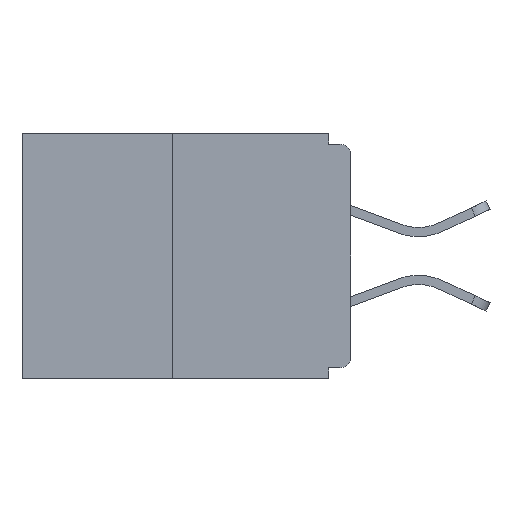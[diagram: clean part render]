
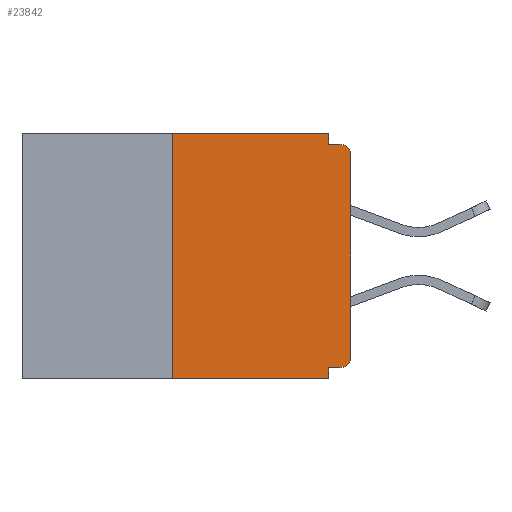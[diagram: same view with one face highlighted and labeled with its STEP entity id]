
A CAD part, left-side view. The second image highlights one B-rep face of the part: STEP entity #23842.
In plain terms, the highlighted planar face has unit normal (-1, 0, 0).
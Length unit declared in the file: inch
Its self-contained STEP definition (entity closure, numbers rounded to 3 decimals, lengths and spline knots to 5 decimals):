
#262 = CARTESIAN_POINT ( 'NONE',  ( 0., 0.015, -0.015 ) ) ;
#579 = CARTESIAN_POINT ( 'NONE',  ( 0., 0.015, -0.328 ) ) ;
#1026 = ORIENTED_EDGE ( 'NONE', *, *, #3591, .F. ) ;
#1222 = VERTEX_POINT ( 'NONE', #15468 ) ;
#1596 = LINE ( 'NONE', #5494, #14856 ) ;
#1816 = EDGE_LOOP ( 'NONE', ( #1026, #21679, #14848, #4472, #8057, #8399, #24403, #12604, #2949, #17886 ) ) ;
#2138 = CARTESIAN_POINT ( 'NONE',  ( 0., 0.031, -0.328 ) ) ;
#2423 = CIRCLE ( 'NONE', #19418, 0.015 ) ;
#2949 = ORIENTED_EDGE ( 'NONE', *, *, #5460, .F. ) ;
#3169 = AXIS2_PLACEMENT_3D ( 'NONE', #14497, #12615, #20066 ) ;
#3219 = CARTESIAN_POINT ( 'NONE',  ( 0., 0.031, -0.343 ) ) ;
#3417 = EDGE_CURVE ( 'NONE', #15087, #22866, #13087, .T. ) ;
#3517 = CARTESIAN_POINT ( 'NONE',  ( 0., 0.25, 0. ) ) ;
#3591 = EDGE_CURVE ( 'NONE', #1222, #23844, #17242, .T. ) ;
#3611 = DIRECTION ( 'NONE',  ( 0., -1., 0. ) ) ;
#3667 = LINE ( 'NONE', #18871, #14287 ) ;
#4472 = ORIENTED_EDGE ( 'NONE', *, *, #3417, .F. ) ;
#4633 = VECTOR ( 'NONE', #23234, 39.37008 ) ;
#5460 = EDGE_CURVE ( 'NONE', #10794, #6925, #3667, .T. ) ;
#5494 = CARTESIAN_POINT ( 'NONE',  ( 0., 0.46, -0.343 ) ) ;
#5943 = CARTESIAN_POINT ( 'NONE',  ( 0., 0.46, 0. ) ) ;
#6136 = VERTEX_POINT ( 'NONE', #579 ) ;
#6344 = EDGE_CURVE ( 'NONE', #21519, #23504, #22492, .T. ) ;
#6925 = VERTEX_POINT ( 'NONE', #262 ) ;
#7069 = EDGE_CURVE ( 'NONE', #23844, #10794, #14672, .T. ) ;
#7860 = CARTESIAN_POINT ( 'NONE',  ( 0., 0., 0. ) ) ;
#8057 = ORIENTED_EDGE ( 'NONE', *, *, #11581, .F. ) ;
#8399 = ORIENTED_EDGE ( 'NONE', *, *, #18187, .T. ) ;
#9705 = LINE ( 'NONE', #3517, #24571 ) ;
#9790 = CARTESIAN_POINT ( 'NONE',  ( 0., 0.031, -0.015 ) ) ;
#10006 = DIRECTION ( 'NONE',  ( -1., 0., 0. ) ) ;
#10794 = VERTEX_POINT ( 'NONE', #9790 ) ;
#11289 = VECTOR ( 'NONE', #23975, 39.37008 ) ;
#11453 = VECTOR ( 'NONE', #12535, 39.37008 ) ;
#11581 = EDGE_CURVE ( 'NONE', #6136, #15087, #17865, .T. ) ;
#11954 = CARTESIAN_POINT ( 'NONE',  ( 0., 0., -0.03 ) ) ;
#12359 = PLANE ( 'NONE',  #3169 ) ;
#12535 = DIRECTION ( 'NONE',  ( 0., 0., -1. ) ) ;
#12558 = DIRECTION ( 'NONE',  ( -1., 0., 0. ) ) ;
#12604 = ORIENTED_EDGE ( 'NONE', *, *, #18115, .T. ) ;
#12615 = DIRECTION ( 'NONE',  ( 1., 0., 0. ) ) ;
#13087 = LINE ( 'NONE', #22949, #11289 ) ;
#13827 = CARTESIAN_POINT ( 'NONE',  ( 0., 0.015, -0.03 ) ) ;
#13964 = CARTESIAN_POINT ( 'NONE',  ( 0., 0., -0.328 ) ) ;
#14156 = CIRCLE ( 'NONE', #23062, 0.015 ) ;
#14212 = EDGE_CURVE ( 'NONE', #14976, #22866, #1596, .T. ) ;
#14284 = CARTESIAN_POINT ( 'NONE',  ( 0., 0.031, 0. ) ) ;
#14287 = VECTOR ( 'NONE', #24703, 39.37008 ) ;
#14497 = CARTESIAN_POINT ( 'NONE',  ( 0., 0.46, 0. ) ) ;
#14571 = DIRECTION ( 'NONE',  ( 0., 0., -1. ) ) ;
#14672 = LINE ( 'NONE', #14284, #11453 ) ;
#14848 = ORIENTED_EDGE ( 'NONE', *, *, #14212, .T. ) ;
#14856 = VECTOR ( 'NONE', #3611, 39.37008 ) ;
#14976 = VERTEX_POINT ( 'NONE', #17101 ) ;
#15087 = VERTEX_POINT ( 'NONE', #2138 ) ;
#15255 = CARTESIAN_POINT ( 'NONE',  ( 0., 0., -0.313 ) ) ;
#15468 = CARTESIAN_POINT ( 'NONE',  ( 0., 0.25, 0. ) ) ;
#17101 = CARTESIAN_POINT ( 'NONE',  ( 0., 0.25, -0.343 ) ) ;
#17242 = LINE ( 'NONE', #5943, #21034 ) ;
#17865 = LINE ( 'NONE', #13964, #4633 ) ;
#17886 = ORIENTED_EDGE ( 'NONE', *, *, #7069, .F. ) ;
#18115 = EDGE_CURVE ( 'NONE', #23504, #6925, #2423, .T. ) ;
#18187 = EDGE_CURVE ( 'NONE', #6136, #21519, #14156, .T. ) ;
#18562 = DIRECTION ( 'NONE',  ( 0., 0., 1. ) ) ;
#18871 = CARTESIAN_POINT ( 'NONE',  ( 0., 0., -0.015 ) ) ;
#19086 = DIRECTION ( 'NONE',  ( 0., 0., 1. ) ) ;
#19161 = VECTOR ( 'NONE', #18562, 39.37008 ) ;
#19400 = DIRECTION ( 'NONE',  ( 0., -1., 0. ) ) ;
#19418 = AXIS2_PLACEMENT_3D ( 'NONE', #13827, #10006, #21788 ) ;
#20066 = DIRECTION ( 'NONE',  ( 0., 0., -1. ) ) ;
#20333 = CARTESIAN_POINT ( 'NONE',  ( 0., 0.031, 0. ) ) ;
#21034 = VECTOR ( 'NONE', #19400, 39.37008 ) ;
#21519 = VERTEX_POINT ( 'NONE', #15255 ) ;
#21679 = ORIENTED_EDGE ( 'NONE', *, *, #24797, .F. ) ;
#21788 = DIRECTION ( 'NONE',  ( 0., 0., -1. ) ) ;
#21974 = FACE_OUTER_BOUND ( 'NONE', #1816, .T. ) ;
#22171 = CARTESIAN_POINT ( 'NONE',  ( 0., 0.015, -0.313 ) ) ;
#22492 = LINE ( 'NONE', #7860, #19161 ) ;
#22866 = VERTEX_POINT ( 'NONE', #3219 ) ;
#22949 = CARTESIAN_POINT ( 'NONE',  ( 0., 0.031, -0.343 ) ) ;
#23062 = AXIS2_PLACEMENT_3D ( 'NONE', #22171, #12558, #14571 ) ;
#23234 = DIRECTION ( 'NONE',  ( 0., 1., 0. ) ) ;
#23504 = VERTEX_POINT ( 'NONE', #11954 ) ;
#23842 = ADVANCED_FACE ( 'NONE', ( #21974 ), #12359, .F. ) ;
#23844 = VERTEX_POINT ( 'NONE', #20333 ) ;
#23975 = DIRECTION ( 'NONE',  ( 0., 0., -1. ) ) ;
#24403 = ORIENTED_EDGE ( 'NONE', *, *, #6344, .T. ) ;
#24571 = VECTOR ( 'NONE', #19086, 39.37008 ) ;
#24703 = DIRECTION ( 'NONE',  ( 0., -1., 0. ) ) ;
#24797 = EDGE_CURVE ( 'NONE', #14976, #1222, #9705, .T. ) ;
